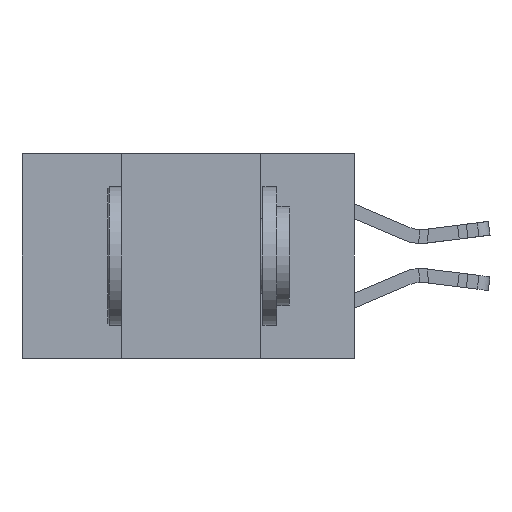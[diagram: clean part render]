
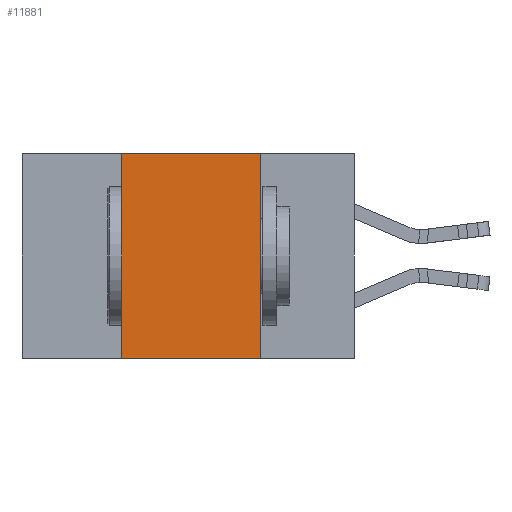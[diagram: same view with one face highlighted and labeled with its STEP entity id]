
A CAD part, left-side view. The second image highlights one B-rep face of the part: STEP entity #11881.
In plain terms, the highlighted planar face has unit normal (-1, 0, 0).
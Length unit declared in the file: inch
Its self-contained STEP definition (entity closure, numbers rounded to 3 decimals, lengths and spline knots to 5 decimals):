
#661 = CARTESIAN_POINT ( 'NONE',  ( 0., 0.6, 0. ) ) ;
#743 = LINE ( 'NONE', #25887, #15147 ) ;
#928 = EDGE_CURVE ( 'NONE', #6437, #16096, #18803, .T. ) ;
#2011 = VERTEX_POINT ( 'NONE', #2525 ) ;
#2525 = CARTESIAN_POINT ( 'NONE',  ( 0., 0.42, 0. ) ) ;
#3847 = VECTOR ( 'NONE', #15832, 39.37008 ) ;
#4062 = CARTESIAN_POINT ( 'NONE',  ( 0., 0.42, -0.37 ) ) ;
#4243 = EDGE_LOOP ( 'NONE', ( #12466, #12192, #19852, #15409 ) ) ;
#5152 = CARTESIAN_POINT ( 'NONE',  ( 0., 0.6, 0. ) ) ;
#6437 = VERTEX_POINT ( 'NONE', #15196 ) ;
#6860 = EDGE_CURVE ( 'NONE', #11665, #16096, #743, .T. ) ;
#7581 = LINE ( 'NONE', #24222, #3847 ) ;
#8695 = DIRECTION ( 'NONE',  ( 0., -1., 0. ) ) ;
#9989 = CARTESIAN_POINT ( 'NONE',  ( 0., 0.17, -0.37 ) ) ;
#11665 = VERTEX_POINT ( 'NONE', #4062 ) ;
#11881 = ADVANCED_FACE ( 'NONE', ( #12460 ), #20857, .F. ) ;
#12192 = ORIENTED_EDGE ( 'NONE', *, *, #20135, .F. ) ;
#12460 = FACE_OUTER_BOUND ( 'NONE', #4243, .T. ) ;
#12466 = ORIENTED_EDGE ( 'NONE', *, *, #928, .F. ) ;
#13163 = CARTESIAN_POINT ( 'NONE',  ( 0., 0.17, -0.37 ) ) ;
#14317 = VECTOR ( 'NONE', #17799, 39.37008 ) ;
#15147 = VECTOR ( 'NONE', #8695, 39.37008 ) ;
#15196 = CARTESIAN_POINT ( 'NONE',  ( 0., 0.17, 0. ) ) ;
#15409 = ORIENTED_EDGE ( 'NONE', *, *, #6860, .T. ) ;
#15492 = DIRECTION ( 'NONE',  ( 0., 0., -1. ) ) ;
#15832 = DIRECTION ( 'NONE',  ( 0., 0., 1. ) ) ;
#16077 = VECTOR ( 'NONE', #16739, 39.37008 ) ;
#16096 = VERTEX_POINT ( 'NONE', #13163 ) ;
#16739 = DIRECTION ( 'NONE',  ( 0., 0., -1. ) ) ;
#17799 = DIRECTION ( 'NONE',  ( 0., -1., 0. ) ) ;
#18803 = LINE ( 'NONE', #9989, #16077 ) ;
#19852 = ORIENTED_EDGE ( 'NONE', *, *, #21964, .F. ) ;
#20135 = EDGE_CURVE ( 'NONE', #2011, #6437, #20358, .T. ) ;
#20358 = LINE ( 'NONE', #5152, #14317 ) ;
#20857 = PLANE ( 'NONE',  #21222 ) ;
#21222 = AXIS2_PLACEMENT_3D ( 'NONE', #661, #21531, #15492 ) ;
#21531 = DIRECTION ( 'NONE',  ( 1., 0., 0. ) ) ;
#21964 = EDGE_CURVE ( 'NONE', #11665, #2011, #7581, .T. ) ;
#24222 = CARTESIAN_POINT ( 'NONE',  ( 0., 0.42, -0.37 ) ) ;
#25887 = CARTESIAN_POINT ( 'NONE',  ( 0., 0.6, -0.37 ) ) ;
